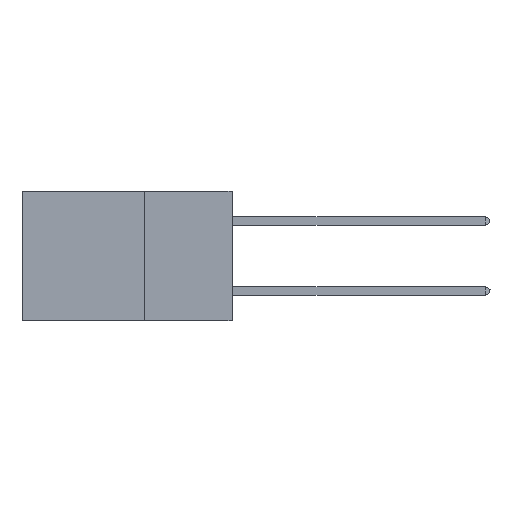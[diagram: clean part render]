
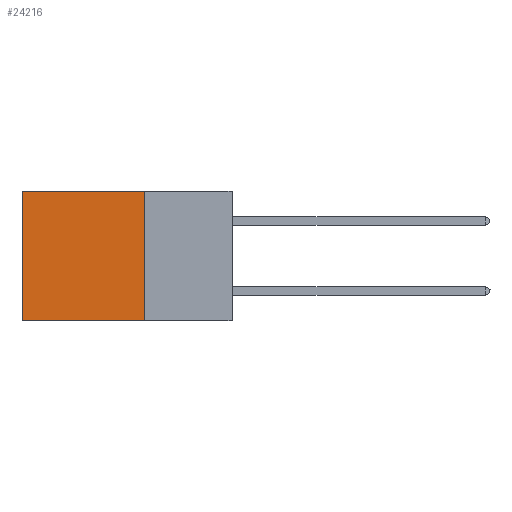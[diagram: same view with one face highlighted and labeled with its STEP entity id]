
A CAD part, left-side view. The second image highlights one B-rep face of the part: STEP entity #24216.
In plain terms, the highlighted planar face has unit normal (-1, 0, 0).
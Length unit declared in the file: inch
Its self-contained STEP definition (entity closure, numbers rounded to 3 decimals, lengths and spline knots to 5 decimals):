
#1609 = CARTESIAN_POINT ( 'NONE',  ( 0.2875, 0.25, -0.37 ) ) ;
#3731 = VERTEX_POINT ( 'NONE', #14650 ) ;
#3787 = EDGE_CURVE ( 'NONE', #10639, #3731, #20505, .T. ) ;
#3918 = VERTEX_POINT ( 'NONE', #15386 ) ;
#4114 = PLANE ( 'NONE',  #14936 ) ;
#5878 = VECTOR ( 'NONE', #24073, 39.37008 ) ;
#7188 = LINE ( 'NONE', #21226, #22908 ) ;
#7223 = VERTEX_POINT ( 'NONE', #1609 ) ;
#8449 = ORIENTED_EDGE ( 'NONE', *, *, #23179, .T. ) ;
#8896 = EDGE_LOOP ( 'NONE', ( #9780, #24559, #29902, #8449 ) ) ;
#9780 = ORIENTED_EDGE ( 'NONE', *, *, #3787, .T. ) ;
#10639 = VERTEX_POINT ( 'NONE', #20953 ) ;
#12290 = DIRECTION ( 'NONE',  ( 0., 1., 0. ) ) ;
#14050 = EDGE_CURVE ( 'NONE', #3918, #7223, #19250, .T. ) ;
#14650 = CARTESIAN_POINT ( 'NONE',  ( 0.2875, 0.6, -0.37 ) ) ;
#14936 = AXIS2_PLACEMENT_3D ( 'NONE', #22810, #20454, #20552 ) ;
#15386 = CARTESIAN_POINT ( 'NONE',  ( 0.2875, 0.25, 0. ) ) ;
#17460 = VECTOR ( 'NONE', #20961, 39.37008 ) ;
#18970 = DIRECTION ( 'NONE',  ( 0., 1., 0. ) ) ;
#19250 = LINE ( 'NONE', #23728, #17460 ) ;
#20454 = DIRECTION ( 'NONE',  ( 1., 0., 0. ) ) ;
#20505 = LINE ( 'NONE', #21615, #5878 ) ;
#20552 = DIRECTION ( 'NONE',  ( 0., 0., -1. ) ) ;
#20953 = CARTESIAN_POINT ( 'NONE',  ( 0.2875, 0.6, 0. ) ) ;
#20961 = DIRECTION ( 'NONE',  ( 0., 0., -1. ) ) ;
#21226 = CARTESIAN_POINT ( 'NONE',  ( 0.2875, 0.25, 0. ) ) ;
#21615 = CARTESIAN_POINT ( 'NONE',  ( 0.2875, 0.6, 0. ) ) ;
#22810 = CARTESIAN_POINT ( 'NONE',  ( 0.2875, 0.25, 0. ) ) ;
#22908 = VECTOR ( 'NONE', #18970, 39.37008 ) ;
#23179 = EDGE_CURVE ( 'NONE', #3918, #10639, #7188, .T. ) ;
#23728 = CARTESIAN_POINT ( 'NONE',  ( 0.2875, 0.25, 0. ) ) ;
#24073 = DIRECTION ( 'NONE',  ( 0., 0., -1. ) ) ;
#24216 = ADVANCED_FACE ( 'NONE', ( #25804 ), #4114, .F. ) ;
#24559 = ORIENTED_EDGE ( 'NONE', *, *, #29048, .F. ) ;
#25804 = FACE_OUTER_BOUND ( 'NONE', #8896, .T. ) ;
#26255 = CARTESIAN_POINT ( 'NONE',  ( 0.2875, 0.25, -0.37 ) ) ;
#28200 = LINE ( 'NONE', #26255, #29282 ) ;
#29048 = EDGE_CURVE ( 'NONE', #7223, #3731, #28200, .T. ) ;
#29282 = VECTOR ( 'NONE', #12290, 39.37008 ) ;
#29902 = ORIENTED_EDGE ( 'NONE', *, *, #14050, .F. ) ;
